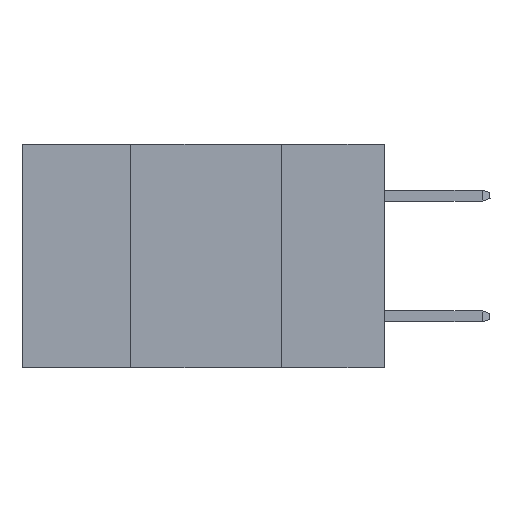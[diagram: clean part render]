
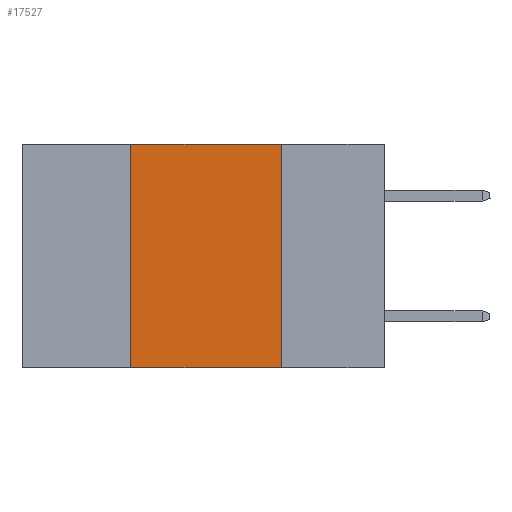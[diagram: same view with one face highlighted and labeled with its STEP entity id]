
A CAD part, left-side view. The second image highlights one B-rep face of the part: STEP entity #17527.
In plain terms, the highlighted planar face has unit normal (-1, 0, 0).
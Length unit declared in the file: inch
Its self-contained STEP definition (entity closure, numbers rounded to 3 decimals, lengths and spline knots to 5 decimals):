
#1083 = LINE ( 'NONE', #12607, #15397 ) ;
#1317 = CARTESIAN_POINT ( 'NONE',  ( 0., 0.17, -0.37 ) ) ;
#2713 = ORIENTED_EDGE ( 'NONE', *, *, #12220, .F. ) ;
#2719 = LINE ( 'NONE', #14874, #10511 ) ;
#2871 = VECTOR ( 'NONE', #4578, 39.37008 ) ;
#3410 = VECTOR ( 'NONE', #5165, 39.37008 ) ;
#3751 = ORIENTED_EDGE ( 'NONE', *, *, #6967, .T. ) ;
#3814 = DIRECTION ( 'NONE',  ( 0., -1., 0. ) ) ;
#3978 = CARTESIAN_POINT ( 'NONE',  ( 0., 0.17, 0. ) ) ;
#4279 = FACE_OUTER_BOUND ( 'NONE', #14831, .T. ) ;
#4578 = DIRECTION ( 'NONE',  ( 0., 0., 1. ) ) ;
#5005 = VERTEX_POINT ( 'NONE', #1317 ) ;
#5165 = DIRECTION ( 'NONE',  ( 0., 0., -1. ) ) ;
#5413 = CARTESIAN_POINT ( 'NONE',  ( 0., 0.6, 0. ) ) ;
#6967 = EDGE_CURVE ( 'NONE', #13789, #5005, #2719, .T. ) ;
#7979 = CARTESIAN_POINT ( 'NONE',  ( 0., 0.17, 0. ) ) ;
#8487 = DIRECTION ( 'NONE',  ( 0., -1., 0. ) ) ;
#8683 = CARTESIAN_POINT ( 'NONE',  ( 0., 0.42, 0. ) ) ;
#9290 = ORIENTED_EDGE ( 'NONE', *, *, #17327, .F. ) ;
#10511 = VECTOR ( 'NONE', #3814, 39.37008 ) ;
#11028 = CARTESIAN_POINT ( 'NONE',  ( 0., 0.42, -0.37 ) ) ;
#11306 = DIRECTION ( 'NONE',  ( 0., 0., -1. ) ) ;
#11406 = VERTEX_POINT ( 'NONE', #3978 ) ;
#11637 = CARTESIAN_POINT ( 'NONE',  ( 0., 0.42, 0. ) ) ;
#12146 = ORIENTED_EDGE ( 'NONE', *, *, #15474, .F. ) ;
#12220 = EDGE_CURVE ( 'NONE', #15525, #11406, #1083, .T. ) ;
#12348 = PLANE ( 'NONE',  #16283 ) ;
#12607 = CARTESIAN_POINT ( 'NONE',  ( 0., 0.6, 0. ) ) ;
#13789 = VERTEX_POINT ( 'NONE', #11028 ) ;
#14831 = EDGE_LOOP ( 'NONE', ( #9290, #2713, #12146, #3751 ) ) ;
#14874 = CARTESIAN_POINT ( 'NONE',  ( 0., 0.6, -0.37 ) ) ;
#15251 = LINE ( 'NONE', #11637, #2871 ) ;
#15397 = VECTOR ( 'NONE', #8487, 39.37008 ) ;
#15474 = EDGE_CURVE ( 'NONE', #13789, #15525, #15251, .T. ) ;
#15525 = VERTEX_POINT ( 'NONE', #8683 ) ;
#15550 = DIRECTION ( 'NONE',  ( 1., 0., 0. ) ) ;
#16283 = AXIS2_PLACEMENT_3D ( 'NONE', #5413, #15550, #11306 ) ;
#17131 = LINE ( 'NONE', #7979, #3410 ) ;
#17327 = EDGE_CURVE ( 'NONE', #11406, #5005, #17131, .T. ) ;
#17527 = ADVANCED_FACE ( 'NONE', ( #4279 ), #12348, .F. ) ;
